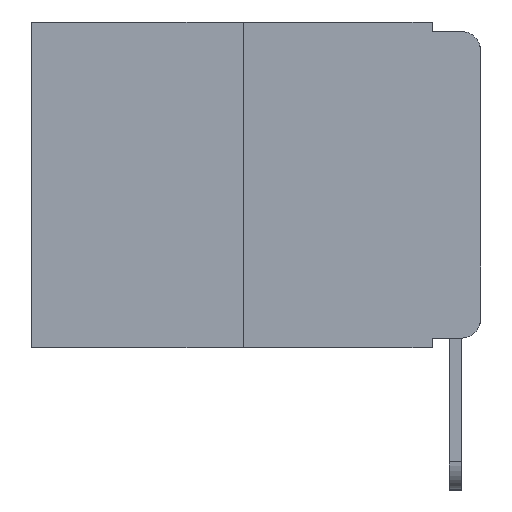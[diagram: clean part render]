
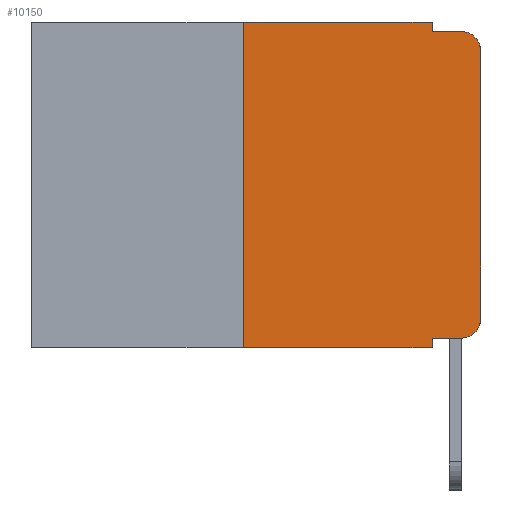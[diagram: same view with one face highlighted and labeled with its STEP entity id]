
A CAD part, left-side view. The second image highlights one B-rep face of the part: STEP entity #10150.
In plain terms, the highlighted planar face has unit normal (-1, 0, 0).
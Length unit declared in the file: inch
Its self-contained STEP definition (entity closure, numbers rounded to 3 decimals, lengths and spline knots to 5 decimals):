
#283 = VERTEX_POINT ( 'NONE', #13640 ) ;
#371 = ORIENTED_EDGE ( 'NONE', *, *, #1465, .T. ) ;
#931 = VERTEX_POINT ( 'NONE', #21432 ) ;
#1465 = EDGE_CURVE ( 'NONE', #13378, #16473, #2855, .T. ) ;
#1502 = DIRECTION ( 'NONE',  ( 0., 0., -1. ) ) ;
#1764 = ORIENTED_EDGE ( 'NONE', *, *, #8249, .T. ) ;
#1933 = ORIENTED_EDGE ( 'NONE', *, *, #13074, .F. ) ;
#1961 = VECTOR ( 'NONE', #8615, 39.37008 ) ;
#2115 = VECTOR ( 'NONE', #3298, 39.37008 ) ;
#2208 = AXIS2_PLACEMENT_3D ( 'NONE', #3265, #9094, #1502 ) ;
#2855 = LINE ( 'NONE', #6183, #5451 ) ;
#3229 = CARTESIAN_POINT ( 'NONE',  ( 0., 0., 0. ) ) ;
#3265 = CARTESIAN_POINT ( 'NONE',  ( 0., 0.02, -0.313 ) ) ;
#3298 = DIRECTION ( 'NONE',  ( 0., 0., 1. ) ) ;
#3356 = EDGE_CURVE ( 'NONE', #13378, #17100, #19733, .T. ) ;
#3544 = DIRECTION ( 'NONE',  ( 0., -1., 0. ) ) ;
#3785 = DIRECTION ( 'NONE',  ( 0., -1., 0. ) ) ;
#4041 = CIRCLE ( 'NONE', #2208, 0.02 ) ;
#4223 = VERTEX_POINT ( 'NONE', #10777 ) ;
#4248 = ORIENTED_EDGE ( 'NONE', *, *, #14830, .F. ) ;
#4434 = CARTESIAN_POINT ( 'NONE',  ( 0., 0.051, 0. ) ) ;
#4505 = LINE ( 'NONE', #6805, #13928 ) ;
#4529 = CARTESIAN_POINT ( 'NONE',  ( 0., 0.25, -0.343 ) ) ;
#4570 = EDGE_CURVE ( 'NONE', #4799, #931, #20952, .T. ) ;
#4705 = PLANE ( 'NONE',  #19722 ) ;
#4799 = VERTEX_POINT ( 'NONE', #16291 ) ;
#5451 = VECTOR ( 'NONE', #6049, 39.37008 ) ;
#5489 = VECTOR ( 'NONE', #16325, 39.37008 ) ;
#5799 = CIRCLE ( 'NONE', #18203, 0.02 ) ;
#6049 = DIRECTION ( 'NONE',  ( 0., -1., 0. ) ) ;
#6129 = EDGE_CURVE ( 'NONE', #283, #9797, #16981, .T. ) ;
#6183 = CARTESIAN_POINT ( 'NONE',  ( 0., 0.473, -0.343 ) ) ;
#6805 = CARTESIAN_POINT ( 'NONE',  ( 0., 0.051, -0.01 ) ) ;
#7720 = VECTOR ( 'NONE', #15599, 39.37008 ) ;
#7838 = DIRECTION ( 'NONE',  ( 1., 0., 0. ) ) ;
#8249 = EDGE_CURVE ( 'NONE', #16705, #9175, #14815, .T. ) ;
#8513 = CARTESIAN_POINT ( 'NONE',  ( 0., 0.051, -0.333 ) ) ;
#8615 = DIRECTION ( 'NONE',  ( 0., 0., -1. ) ) ;
#9094 = DIRECTION ( 'NONE',  ( -1., 0., 0. ) ) ;
#9175 = VERTEX_POINT ( 'NONE', #14616 ) ;
#9530 = DIRECTION ( 'NONE',  ( 0., 0., -1. ) ) ;
#9797 = VERTEX_POINT ( 'NONE', #10138 ) ;
#10138 = CARTESIAN_POINT ( 'NONE',  ( 0., 0., -0.03 ) ) ;
#10150 = ADVANCED_FACE ( 'NONE', ( #12363 ), #4705, .F. ) ;
#10374 = ORIENTED_EDGE ( 'NONE', *, *, #6129, .T. ) ;
#10777 = CARTESIAN_POINT ( 'NONE',  ( 0., 0.02, -0.01 ) ) ;
#11162 = ORIENTED_EDGE ( 'NONE', *, *, #4570, .F. ) ;
#12022 = LINE ( 'NONE', #13270, #5489 ) ;
#12238 = CARTESIAN_POINT ( 'NONE',  ( 0., 0.25, 0. ) ) ;
#12363 = FACE_OUTER_BOUND ( 'NONE', #21112, .T. ) ;
#12703 = EDGE_CURVE ( 'NONE', #9797, #4223, #5799, .T. ) ;
#13074 = EDGE_CURVE ( 'NONE', #931, #4223, #4505, .T. ) ;
#13076 = CARTESIAN_POINT ( 'NONE',  ( 0., 0.051, -0.343 ) ) ;
#13270 = CARTESIAN_POINT ( 'NONE',  ( 0., 0.473, 0. ) ) ;
#13378 = VERTEX_POINT ( 'NONE', #4529 ) ;
#13640 = CARTESIAN_POINT ( 'NONE',  ( 0., 0., -0.313 ) ) ;
#13833 = DIRECTION ( 'NONE',  ( -1., 0., 0. ) ) ;
#13907 = DIRECTION ( 'NONE',  ( 0., 0., -1. ) ) ;
#13928 = VECTOR ( 'NONE', #3544, 39.37008 ) ;
#14096 = LINE ( 'NONE', #4434, #18503 ) ;
#14184 = EDGE_CURVE ( 'NONE', #17100, #4799, #12022, .T. ) ;
#14223 = CARTESIAN_POINT ( 'NONE',  ( 0., 0.25, 0. ) ) ;
#14616 = CARTESIAN_POINT ( 'NONE',  ( 0., 0.02, -0.333 ) ) ;
#14815 = LINE ( 'NONE', #8513, #15343 ) ;
#14830 = EDGE_CURVE ( 'NONE', #16705, #16473, #14096, .T. ) ;
#15343 = VECTOR ( 'NONE', #3785, 39.37008 ) ;
#15364 = ORIENTED_EDGE ( 'NONE', *, *, #15740, .T. ) ;
#15599 = DIRECTION ( 'NONE',  ( 0., 0., 1. ) ) ;
#15740 = EDGE_CURVE ( 'NONE', #9175, #283, #4041, .T. ) ;
#16291 = CARTESIAN_POINT ( 'NONE',  ( 0., 0.051, 0. ) ) ;
#16325 = DIRECTION ( 'NONE',  ( 0., -1., 0. ) ) ;
#16473 = VERTEX_POINT ( 'NONE', #13076 ) ;
#16705 = VERTEX_POINT ( 'NONE', #20486 ) ;
#16774 = ORIENTED_EDGE ( 'NONE', *, *, #12703, .T. ) ;
#16981 = LINE ( 'NONE', #3229, #2115 ) ;
#17100 = VERTEX_POINT ( 'NONE', #14223 ) ;
#17855 = DIRECTION ( 'NONE',  ( 0., 0., -1. ) ) ;
#18203 = AXIS2_PLACEMENT_3D ( 'NONE', #20503, #13833, #13907 ) ;
#18503 = VECTOR ( 'NONE', #17855, 39.37008 ) ;
#18628 = CARTESIAN_POINT ( 'NONE',  ( 0., 0.051, 0. ) ) ;
#19517 = CARTESIAN_POINT ( 'NONE',  ( 0., 0.473, 0. ) ) ;
#19722 = AXIS2_PLACEMENT_3D ( 'NONE', #19517, #7838, #9530 ) ;
#19733 = LINE ( 'NONE', #12238, #7720 ) ;
#20486 = CARTESIAN_POINT ( 'NONE',  ( 0., 0.051, -0.333 ) ) ;
#20503 = CARTESIAN_POINT ( 'NONE',  ( 0., 0.02, -0.03 ) ) ;
#20713 = ORIENTED_EDGE ( 'NONE', *, *, #14184, .F. ) ;
#20843 = ORIENTED_EDGE ( 'NONE', *, *, #3356, .F. ) ;
#20952 = LINE ( 'NONE', #18628, #1961 ) ;
#21112 = EDGE_LOOP ( 'NONE', ( #10374, #16774, #1933, #11162, #20713, #20843, #371, #4248, #1764, #15364 ) ) ;
#21432 = CARTESIAN_POINT ( 'NONE',  ( 0., 0.051, -0.01 ) ) ;
